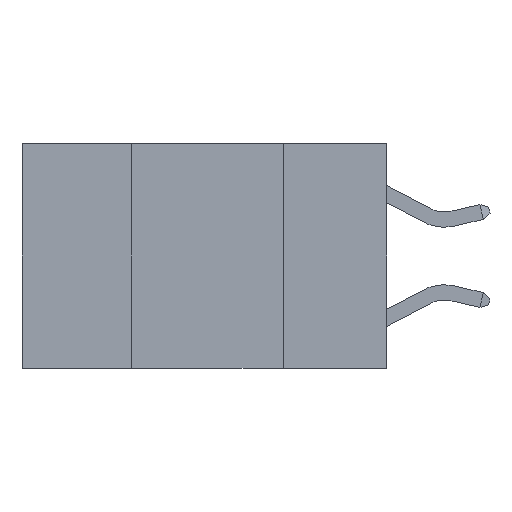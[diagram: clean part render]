
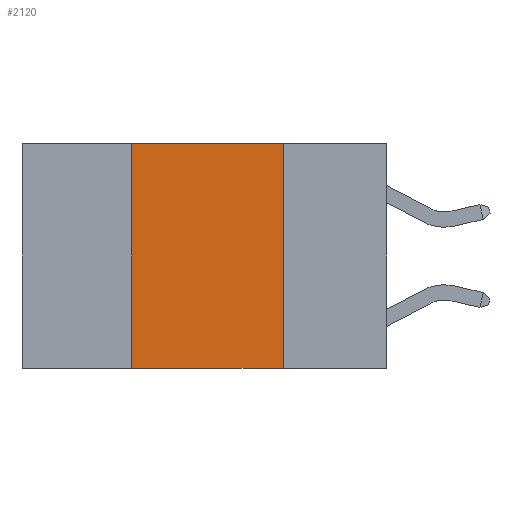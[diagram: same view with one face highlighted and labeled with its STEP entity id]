
A CAD part, left-side view. The second image highlights one B-rep face of the part: STEP entity #2120.
In plain terms, the highlighted planar face has unit normal (-1, 0, 0).
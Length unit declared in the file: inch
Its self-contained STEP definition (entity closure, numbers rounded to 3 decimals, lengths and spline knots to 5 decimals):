
#73 = DIRECTION ( 'NONE',  ( 0., 0., 1. ) ) ;
#132 = VERTEX_POINT ( 'NONE', #5479 ) ;
#506 = VERTEX_POINT ( 'NONE', #8814 ) ;
#1375 = EDGE_LOOP ( 'NONE', ( #4803, #4926, #5199, #5665 ) ) ;
#1536 = CARTESIAN_POINT ( 'NONE',  ( 0., 0.6, 0. ) ) ;
#1709 = EDGE_CURVE ( 'NONE', #5332, #132, #4429, .T. ) ;
#2042 = CARTESIAN_POINT ( 'NONE',  ( 0., 0.42, 0. ) ) ;
#2120 = ADVANCED_FACE ( 'NONE', ( #5566 ), #11807, .F. ) ;
#2600 = DIRECTION ( 'NONE',  ( 0., -1., 0. ) ) ;
#2880 = AXIS2_PLACEMENT_3D ( 'NONE', #1536, #11592, #11496 ) ;
#3044 = EDGE_CURVE ( 'NONE', #5332, #506, #4398, .T. ) ;
#3517 = CARTESIAN_POINT ( 'NONE',  ( 0., 0.6, 0. ) ) ;
#4057 = LINE ( 'NONE', #8070, #10989 ) ;
#4398 = LINE ( 'NONE', #2042, #11312 ) ;
#4429 = LINE ( 'NONE', #9170, #8994 ) ;
#4803 = ORIENTED_EDGE ( 'NONE', *, *, #5258, .F. ) ;
#4926 = ORIENTED_EDGE ( 'NONE', *, *, #8988, .F. ) ;
#5199 = ORIENTED_EDGE ( 'NONE', *, *, #3044, .F. ) ;
#5258 = EDGE_CURVE ( 'NONE', #11232, #132, #4057, .T. ) ;
#5332 = VERTEX_POINT ( 'NONE', #5651 ) ;
#5479 = CARTESIAN_POINT ( 'NONE',  ( 0., 0.17, -0.37 ) ) ;
#5566 = FACE_OUTER_BOUND ( 'NONE', #1375, .T. ) ;
#5651 = CARTESIAN_POINT ( 'NONE',  ( 0., 0.42, -0.37 ) ) ;
#5665 = ORIENTED_EDGE ( 'NONE', *, *, #1709, .T. ) ;
#6512 = VECTOR ( 'NONE', #2600, 39.37008 ) ;
#6821 = LINE ( 'NONE', #3517, #6512 ) ;
#7653 = CARTESIAN_POINT ( 'NONE',  ( 0., 0.17, 0. ) ) ;
#8070 = CARTESIAN_POINT ( 'NONE',  ( 0., 0.17, 0. ) ) ;
#8659 = DIRECTION ( 'NONE',  ( 0., -1., 0. ) ) ;
#8814 = CARTESIAN_POINT ( 'NONE',  ( 0., 0.42, 0. ) ) ;
#8988 = EDGE_CURVE ( 'NONE', #506, #11232, #6821, .T. ) ;
#8994 = VECTOR ( 'NONE', #8659, 39.37008 ) ;
#9170 = CARTESIAN_POINT ( 'NONE',  ( 0., 0.6, -0.37 ) ) ;
#10989 = VECTOR ( 'NONE', #11598, 39.37008 ) ;
#11232 = VERTEX_POINT ( 'NONE', #7653 ) ;
#11312 = VECTOR ( 'NONE', #73, 39.37008 ) ;
#11496 = DIRECTION ( 'NONE',  ( 0., 0., -1. ) ) ;
#11592 = DIRECTION ( 'NONE',  ( 1., 0., 0. ) ) ;
#11598 = DIRECTION ( 'NONE',  ( 0., 0., -1. ) ) ;
#11807 = PLANE ( 'NONE',  #2880 ) ;
